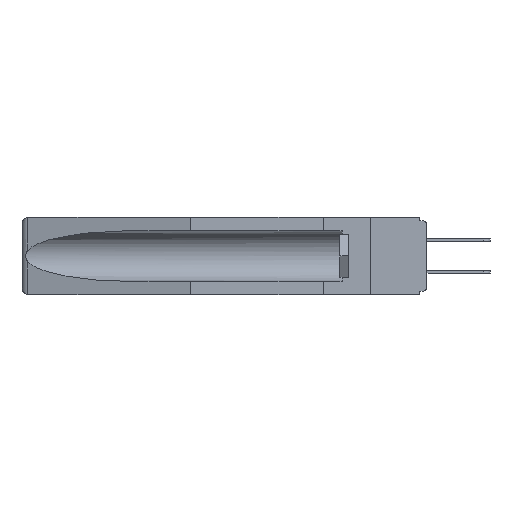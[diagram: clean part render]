
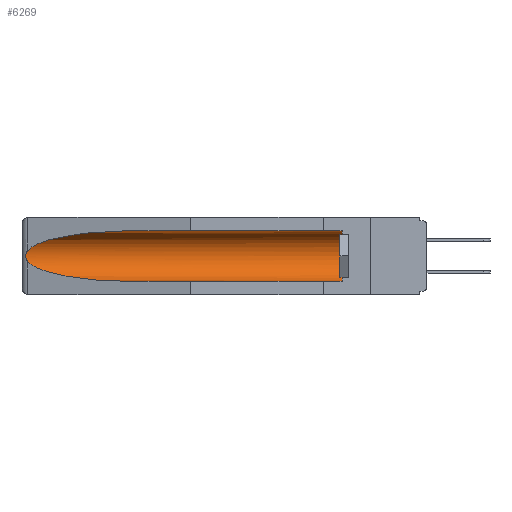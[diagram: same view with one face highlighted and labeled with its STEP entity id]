
A CAD part, left-side view. The second image highlights one B-rep face of the part: STEP entity #6269.
In plain terms, the highlighted cylindrical face has radius 2.857 mm (diameter 5.715 mm), a partial arc.
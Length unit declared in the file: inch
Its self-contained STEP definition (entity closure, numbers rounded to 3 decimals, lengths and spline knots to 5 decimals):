
#13 = EDGE_CURVE ( 'NONE', #16928, #11073, #17133, .T. ) ;
#77 = CARTESIAN_POINT ( 'NONE',  ( 0.26597, 1.5296, -0.19026 ) ) ;
#653 = CYLINDRICAL_SURFACE ( 'NONE', #11141, 0.1125 ) ;
#694 = EDGE_CURVE ( 'NONE', #3687, #16543, #806, .T. ) ;
#806 = LINE ( 'NONE', #9379, #19709 ) ;
#861 = CARTESIAN_POINT ( 'NONE',  ( 0.21114, 1.30732, -0.284 ) ) ;
#1139 = CARTESIAN_POINT ( 'NONE',  ( 0.26537, 1.52718, -0.19328 ) ) ;
#1699 = ORIENTED_EDGE ( 'NONE', *, *, #13, .T. ) ;
#1798 = CARTESIAN_POINT ( 'NONE',  ( 0.2675, 1.53308, -0.16763 ) ) ;
#3063 = DIRECTION ( 'NONE',  ( 0., 0., 1. ) ) ;
#3294 = EDGE_LOOP ( 'NONE', ( #12138, #1699, #9209, #14234, #11532, #8078 ) ) ;
#3687 = VERTEX_POINT ( 'NONE', #19274 ) ;
#3980 = EDGE_CURVE ( 'NONE', #16543, #16928, #6141, .T. ) ;
#4015 = CIRCLE ( 'NONE', #9837, 0.1125 ) ;
#4447 = DIRECTION ( 'NONE',  ( 0., 0., 1. ) ) ;
#4634 = CARTESIAN_POINT ( 'NONE',  ( 0.155, 0.126, -0.284 ) ) ;
#4791 = CARTESIAN_POINT ( 'NONE',  ( 0.2673, 1.53269, -0.17917 ) ) ;
#5137 =( BOUNDED_CURVE ( )  B_SPLINE_CURVE ( 3, ( #1139, #14795, #861, #5519 ),
 .UNSPECIFIED., .F., .F. ) 
 B_SPLINE_CURVE_WITH_KNOTS ( ( 4, 4 ),
 ( 0.1948, 1.5708 ),
 .UNSPECIFIED. ) 
 CURVE ( )  GEOMETRIC_REPRESENTATION_ITEM ( )  RATIONAL_B_SPLINE_CURVE ( ( 1., 0.848, 0.848, 1. ) ) 
 REPRESENTATION_ITEM ( '' )  );
#5519 = CARTESIAN_POINT ( 'NONE',  ( 0.155, 1.07973, -0.284 ) ) ;
#5956 = CARTESIAN_POINT ( 'NONE',  ( 0.25451, 1.48313, -0.09465 ) ) ;
#6141 =( BOUNDED_CURVE ( )  B_SPLINE_CURVE ( 3, ( #8929, #9064, #5956, #19848 ),
 .UNSPECIFIED., .F., .F. ) 
 B_SPLINE_CURVE_WITH_KNOTS ( ( 4, 4 ),
 ( 4.71239, 6.08839 ),
 .UNSPECIFIED. ) 
 CURVE ( )  GEOMETRIC_REPRESENTATION_ITEM ( )  RATIONAL_B_SPLINE_CURVE ( ( 1., 0.848, 0.848, 1. ) ) 
 REPRESENTATION_ITEM ( '' )  );
#6209 = CARTESIAN_POINT ( 'NONE',  ( 0.26537, 1.52718, -0.19328 ) ) ;
#6269 = ADVANCED_FACE ( 'NONE', ( #13068 ), #653, .F. ) ;
#6521 = CARTESIAN_POINT ( 'NONE',  ( 0.26655, 1.53094, -0.18657 ) ) ;
#7062 = EDGE_CURVE ( 'NONE', #10611, #11126, #17346, .T. ) ;
#7774 = CARTESIAN_POINT ( 'NONE',  ( 0.155, 1.07973, -0.284 ) ) ;
#8078 = ORIENTED_EDGE ( 'NONE', *, *, #694, .T. ) ;
#8880 = CARTESIAN_POINT ( 'NONE',  ( 0.155, -0.30754, -0.1715 ) ) ;
#8929 = CARTESIAN_POINT ( 'NONE',  ( 0.155, 1.07973, -0.059 ) ) ;
#9064 = CARTESIAN_POINT ( 'NONE',  ( 0.21114, 1.30732, -0.059 ) ) ;
#9127 = CARTESIAN_POINT ( 'NONE',  ( 0.155, 1.07973, -0.059 ) ) ;
#9209 = ORIENTED_EDGE ( 'NONE', *, *, #19545, .T. ) ;
#9379 = CARTESIAN_POINT ( 'NONE',  ( 0.155, -0.30754, -0.059 ) ) ;
#9837 = AXIS2_PLACEMENT_3D ( 'NONE', #12114, #19916, #3063 ) ;
#10611 = VERTEX_POINT ( 'NONE', #4634 ) ;
#11073 = VERTEX_POINT ( 'NONE', #6209 ) ;
#11126 = VERTEX_POINT ( 'NONE', #7774 ) ;
#11141 = AXIS2_PLACEMENT_3D ( 'NONE', #8880, #14021, #4447 ) ;
#11532 = ORIENTED_EDGE ( 'NONE', *, *, #14158, .T. ) ;
#11966 = DIRECTION ( 'NONE',  ( 0., 1., 0. ) ) ;
#12114 = CARTESIAN_POINT ( 'NONE',  ( 0.155, 0.126, -0.1715 ) ) ;
#12138 = ORIENTED_EDGE ( 'NONE', *, *, #3980, .T. ) ;
#12598 = CARTESIAN_POINT ( 'NONE',  ( 0.26537, 1.52718, -0.19328 ) ) ;
#13068 = FACE_OUTER_BOUND ( 'NONE', #3294, .T. ) ;
#14021 = DIRECTION ( 'NONE',  ( 0., 1., 0. ) ) ;
#14106 = CARTESIAN_POINT ( 'NONE',  ( 0.26597, 1.52961, -0.15275 ) ) ;
#14158 = EDGE_CURVE ( 'NONE', #10611, #3687, #4015, .T. ) ;
#14234 = ORIENTED_EDGE ( 'NONE', *, *, #7062, .F. ) ;
#14242 = CARTESIAN_POINT ( 'NONE',  ( 0.2673, 1.5327, -0.16383 ) ) ;
#14795 = CARTESIAN_POINT ( 'NONE',  ( 0.25451, 1.48313, -0.24835 ) ) ;
#15777 = CARTESIAN_POINT ( 'NONE',  ( 0.2675, 1.53308, -0.17534 ) ) ;
#16543 = VERTEX_POINT ( 'NONE', #9127 ) ;
#16856 = VECTOR ( 'NONE', #11966, 39.37008 ) ;
#16919 = DIRECTION ( 'NONE',  ( 0., 1., 0. ) ) ;
#16928 = VERTEX_POINT ( 'NONE', #17257 ) ;
#17133 = B_SPLINE_CURVE_WITH_KNOTS ( 'NONE', 3,
 ( #18773, #14106, #17357, #14242, #1798, #15777, #4791, #6521, #77, #12598 ),
 .UNSPECIFIED., .F., .F.,
 ( 4, 2, 2, 2, 4 ),
 ( 0., 0.00029, 0.00058, 0.00087, 0.00117 ),
 .UNSPECIFIED. ) ;
#17257 = CARTESIAN_POINT ( 'NONE',  ( 0.26537, 1.52718, -0.14972 ) ) ;
#17346 = LINE ( 'NONE', #19630, #16856 ) ;
#17357 = CARTESIAN_POINT ( 'NONE',  ( 0.26654, 1.53092, -0.15636 ) ) ;
#18773 = CARTESIAN_POINT ( 'NONE',  ( 0.26537, 1.52718, -0.14972 ) ) ;
#19274 = CARTESIAN_POINT ( 'NONE',  ( 0.155, 0.126, -0.059 ) ) ;
#19545 = EDGE_CURVE ( 'NONE', #11073, #11126, #5137, .T. ) ;
#19630 = CARTESIAN_POINT ( 'NONE',  ( 0.155, -0.30754, -0.284 ) ) ;
#19709 = VECTOR ( 'NONE', #16919, 39.37008 ) ;
#19848 = CARTESIAN_POINT ( 'NONE',  ( 0.26537, 1.52718, -0.14972 ) ) ;
#19916 = DIRECTION ( 'NONE',  ( 0., -1., 0. ) ) ;
